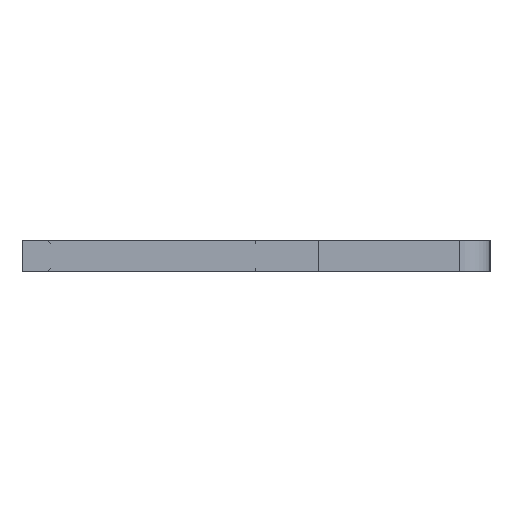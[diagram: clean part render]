
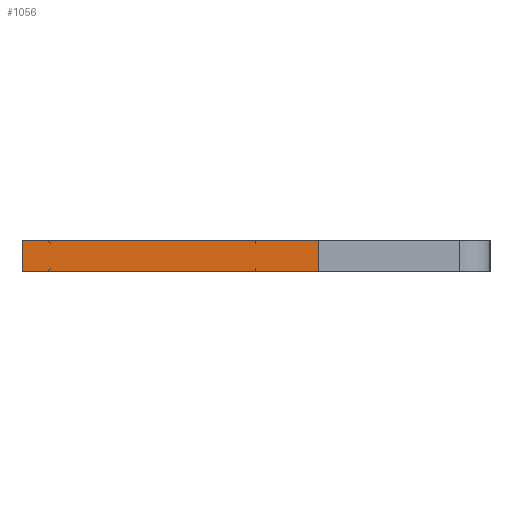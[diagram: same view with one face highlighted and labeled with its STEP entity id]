
A CAD part, left-side view. The second image highlights one B-rep face of the part: STEP entity #1056.
In plain terms, the highlighted face is planar.
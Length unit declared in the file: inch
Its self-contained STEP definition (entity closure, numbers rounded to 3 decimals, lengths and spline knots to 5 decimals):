
#27 = VERTEX_POINT ( 'NONE', #1696 ) ;
#158 = DIRECTION ( 'NONE',  ( 0., 0., 1. ) ) ;
#180 = VECTOR ( 'NONE', #1481, 39.37008 ) ;
#204 = VERTEX_POINT ( 'NONE', #1884 ) ;
#215 = DIRECTION ( 'NONE',  ( 0., 1., 0. ) ) ;
#239 = LINE ( 'NONE', #1358, #1571 ) ;
#279 = VERTEX_POINT ( 'NONE', #566 ) ;
#331 = CARTESIAN_POINT ( 'NONE',  ( 0.01, 0.15, -0.04 ) ) ;
#528 = CARTESIAN_POINT ( 'NONE',  ( -0.01, 0.15, -0.04 ) ) ;
#566 = CARTESIAN_POINT ( 'NONE',  ( 0.01, -0.04, -0.04 ) ) ;
#578 = ORIENTED_EDGE ( 'NONE', *, *, #903, .F. ) ;
#614 = ORIENTED_EDGE ( 'NONE', *, *, #1610, .T. ) ;
#619 = ORIENTED_EDGE ( 'NONE', *, *, #921, .T. ) ;
#667 = LINE ( 'NONE', #989, #956 ) ;
#773 = EDGE_LOOP ( 'NONE', ( #614, #1552, #578, #619 ) ) ;
#809 = CARTESIAN_POINT ( 'NONE',  ( 0.01, -0.04, -0.04 ) ) ;
#903 = EDGE_CURVE ( 'NONE', #279, #27, #1043, .T. ) ;
#921 = EDGE_CURVE ( 'NONE', #279, #204, #1502, .T. ) ;
#956 = VECTOR ( 'NONE', #215, 39.37008 ) ;
#989 = CARTESIAN_POINT ( 'NONE',  ( -0.01, 0.15, -0.04 ) ) ;
#1043 = LINE ( 'NONE', #331, #180 ) ;
#1056 = ADVANCED_FACE ( 'NONE', ( #1145 ), #1988, .F. ) ;
#1145 = FACE_OUTER_BOUND ( 'NONE', #773, .T. ) ;
#1306 = DIRECTION ( 'NONE',  ( 1., 0., 0. ) ) ;
#1316 = DIRECTION ( 'NONE',  ( -1., 0., 0. ) ) ;
#1358 = CARTESIAN_POINT ( 'NONE',  ( 0.01, 0.15, -0.04 ) ) ;
#1396 = EDGE_CURVE ( 'NONE', #27, #1882, #239, .T. ) ;
#1454 = VECTOR ( 'NONE', #1316, 39.37008 ) ;
#1481 = DIRECTION ( 'NONE',  ( 0., 1., 0. ) ) ;
#1502 = LINE ( 'NONE', #809, #1454 ) ;
#1552 = ORIENTED_EDGE ( 'NONE', *, *, #1396, .F. ) ;
#1571 = VECTOR ( 'NONE', #1854, 39.37008 ) ;
#1610 = EDGE_CURVE ( 'NONE', #204, #1882, #667, .T. ) ;
#1696 = CARTESIAN_POINT ( 'NONE',  ( 0.01, 0.15, -0.04 ) ) ;
#1854 = DIRECTION ( 'NONE',  ( -1., 0., 0. ) ) ;
#1882 = VERTEX_POINT ( 'NONE', #528 ) ;
#1884 = CARTESIAN_POINT ( 'NONE',  ( -0.01, -0.04, -0.04 ) ) ;
#1988 = PLANE ( 'NONE',  #1990 ) ;
#1990 = AXIS2_PLACEMENT_3D ( 'NONE', #1996, #158, #1306 ) ;
#1996 = CARTESIAN_POINT ( 'NONE',  ( 0.01, 0.15, -0.04 ) ) ;
